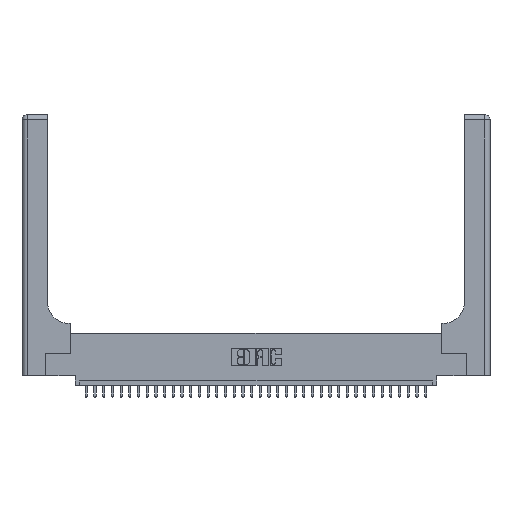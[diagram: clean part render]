
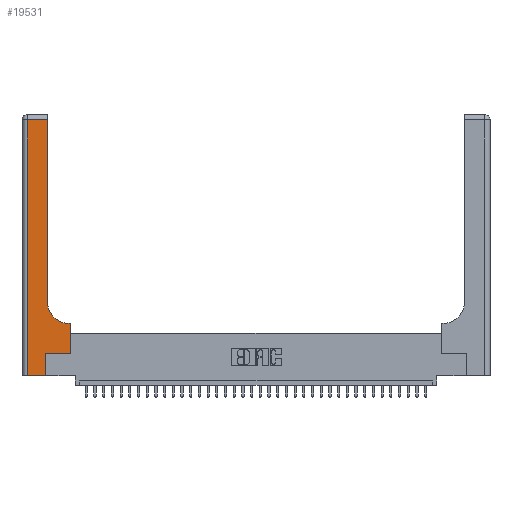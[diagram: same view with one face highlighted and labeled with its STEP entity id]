
A CAD part, top view. The second image highlights one B-rep face of the part: STEP entity #19531.
In plain terms, the highlighted planar face has unit normal (0, 0, 1).
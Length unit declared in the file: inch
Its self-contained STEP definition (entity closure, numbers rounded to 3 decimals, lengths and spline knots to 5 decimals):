
#1091 = EDGE_CURVE ( 'NONE', #22268, #33041, #28709, .T. ) ;
#1262 = VERTEX_POINT ( 'NONE', #17304 ) ;
#1428 = CARTESIAN_POINT ( 'NONE',  ( 0., 2.94, 0.37 ) ) ;
#1882 = ORIENTED_EDGE ( 'NONE', *, *, #11492, .T. ) ;
#2003 = DIRECTION ( 'NONE',  ( 1., 0., 0. ) ) ;
#3401 = ORIENTED_EDGE ( 'NONE', *, *, #23466, .T. ) ;
#3465 = LINE ( 'NONE', #20936, #10047 ) ;
#3834 = VERTEX_POINT ( 'NONE', #18381 ) ;
#3891 = CARTESIAN_POINT ( 'NONE',  ( 0.2915, 2.94, 0.37 ) ) ;
#4632 = LINE ( 'NONE', #24647, #20209 ) ;
#5099 = CARTESIAN_POINT ( 'NONE',  ( 0.2915, 0.6, 0.37 ) ) ;
#5319 = CARTESIAN_POINT ( 'NONE',  ( 0.269, 0.25, 0.37 ) ) ;
#5358 = VECTOR ( 'NONE', #32381, 39.37008 ) ;
#5665 = CARTESIAN_POINT ( 'NONE',  ( 0.5415, 0.85, 0.37 ) ) ;
#6366 = DIRECTION ( 'NONE',  ( 0., 1., 0. ) ) ;
#6509 = ORIENTED_EDGE ( 'NONE', *, *, #30265, .T. ) ;
#6642 = VECTOR ( 'NONE', #2003, 39.37008 ) ;
#8157 = ORIENTED_EDGE ( 'NONE', *, *, #1091, .T. ) ;
#8181 = LINE ( 'NONE', #26096, #28896 ) ;
#8448 = LINE ( 'NONE', #5319, #5358 ) ;
#9650 = DIRECTION ( 'NONE',  ( -1., 0., 0. ) ) ;
#9941 = LINE ( 'NONE', #5099, #31066 ) ;
#9994 = CARTESIAN_POINT ( 'NONE',  ( 0.269, 0.25, 0.37 ) ) ;
#10047 = VECTOR ( 'NONE', #10195, 39.37008 ) ;
#10195 = DIRECTION ( 'NONE',  ( 0., -1., 0. ) ) ;
#10481 = DIRECTION ( 'NONE',  ( -1., 0., 0. ) ) ;
#10537 = EDGE_CURVE ( 'NONE', #33041, #14741, #4632, .T. ) ;
#11492 = EDGE_CURVE ( 'NONE', #14741, #24586, #22607, .T. ) ;
#12146 = CARTESIAN_POINT ( 'NONE',  ( 0.5585, 0.25, 0.37 ) ) ;
#13148 = EDGE_CURVE ( 'NONE', #24586, #20225, #3465, .T. ) ;
#13354 = CARTESIAN_POINT ( 'NONE',  ( 0., 3., 0.37 ) ) ;
#13826 = CARTESIAN_POINT ( 'NONE',  ( 0.5415, 0.6, 0.37 ) ) ;
#13992 = ORIENTED_EDGE ( 'NONE', *, *, #13148, .T. ) ;
#14533 = FACE_OUTER_BOUND ( 'NONE', #28985, .T. ) ;
#14552 = DIRECTION ( 'NONE',  ( 0., 1., 0. ) ) ;
#14741 = VERTEX_POINT ( 'NONE', #3891 ) ;
#15440 = CARTESIAN_POINT ( 'NONE',  ( 0.06, 0., 0.37 ) ) ;
#15792 = PLANE ( 'NONE',  #26242 ) ;
#16479 = DIRECTION ( 'NONE',  ( 1., 0., 0. ) ) ;
#16520 = VECTOR ( 'NONE', #9650, 39.37008 ) ;
#17304 = CARTESIAN_POINT ( 'NONE',  ( 0.5585, 0.6, 0.37 ) ) ;
#17462 = DIRECTION ( 'NONE',  ( 0., 1., 0. ) ) ;
#18279 = CARTESIAN_POINT ( 'NONE',  ( 0., 0., 0.37 ) ) ;
#18381 = CARTESIAN_POINT ( 'NONE',  ( 0.269, 0., 0.37 ) ) ;
#18915 = DIRECTION ( 'NONE',  ( -1., 0., 0. ) ) ;
#19406 = ORIENTED_EDGE ( 'NONE', *, *, #31084, .T. ) ;
#19531 = ADVANCED_FACE ( 'NONE', ( #14533 ), #15792, .F. ) ;
#20209 = VECTOR ( 'NONE', #14552, 39.37008 ) ;
#20225 = VERTEX_POINT ( 'NONE', #15440 ) ;
#20936 = CARTESIAN_POINT ( 'NONE',  ( 0.06, 3., 0.37 ) ) ;
#21580 = CARTESIAN_POINT ( 'NONE',  ( 0.5585, 0.25, 0.37 ) ) ;
#22268 = VERTEX_POINT ( 'NONE', #13826 ) ;
#22607 = LINE ( 'NONE', #1428, #16520 ) ;
#23466 = EDGE_CURVE ( 'NONE', #1262, #22268, #9941, .T. ) ;
#24000 = DIRECTION ( 'NONE',  ( 0., 0., -1. ) ) ;
#24155 = LINE ( 'NONE', #12146, #34883 ) ;
#24586 = VERTEX_POINT ( 'NONE', #33446 ) ;
#24647 = CARTESIAN_POINT ( 'NONE',  ( 0.2915, 3., 0.37 ) ) ;
#25453 = VERTEX_POINT ( 'NONE', #9994 ) ;
#26096 = CARTESIAN_POINT ( 'NONE',  ( 0.269, 0., 0.37 ) ) ;
#26242 = AXIS2_PLACEMENT_3D ( 'NONE', #13354, #24000, #10481 ) ;
#26898 = ORIENTED_EDGE ( 'NONE', *, *, #33304, .T. ) ;
#27806 = DIRECTION ( 'NONE',  ( 0., 0., -1. ) ) ;
#28709 = CIRCLE ( 'NONE', #33168, 0.25 ) ;
#28896 = VECTOR ( 'NONE', #6366, 39.37008 ) ;
#28985 = EDGE_LOOP ( 'NONE', ( #29196, #1882, #13992, #26898, #19406, #33092, #6509, #3401, #8157 ) ) ;
#29196 = ORIENTED_EDGE ( 'NONE', *, *, #10537, .T. ) ;
#30265 = EDGE_CURVE ( 'NONE', #35669, #1262, #24155, .T. ) ;
#31007 = CARTESIAN_POINT ( 'NONE',  ( 0.2915, 0.85, 0.37 ) ) ;
#31066 = VECTOR ( 'NONE', #18915, 39.37008 ) ;
#31084 = EDGE_CURVE ( 'NONE', #3834, #25453, #8181, .T. ) ;
#32381 = DIRECTION ( 'NONE',  ( 1., 0., 0. ) ) ;
#32933 = EDGE_CURVE ( 'NONE', #25453, #35669, #8448, .T. ) ;
#33041 = VERTEX_POINT ( 'NONE', #31007 ) ;
#33092 = ORIENTED_EDGE ( 'NONE', *, *, #32933, .T. ) ;
#33168 = AXIS2_PLACEMENT_3D ( 'NONE', #5665, #27806, #16479 ) ;
#33304 = EDGE_CURVE ( 'NONE', #20225, #3834, #35150, .T. ) ;
#33446 = CARTESIAN_POINT ( 'NONE',  ( 0.06, 2.94, 0.37 ) ) ;
#34883 = VECTOR ( 'NONE', #17462, 39.37008 ) ;
#35150 = LINE ( 'NONE', #18279, #6642 ) ;
#35669 = VERTEX_POINT ( 'NONE', #21580 ) ;
